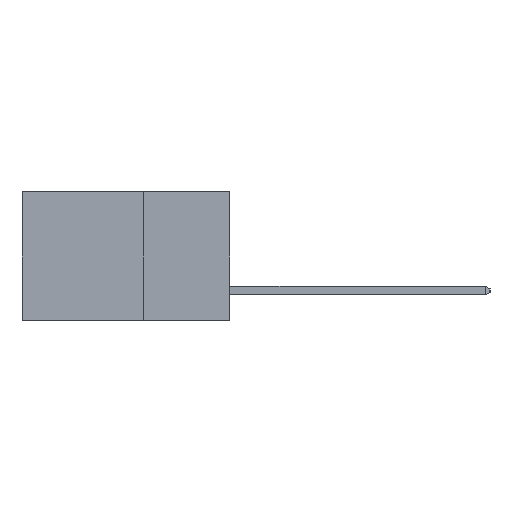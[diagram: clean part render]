
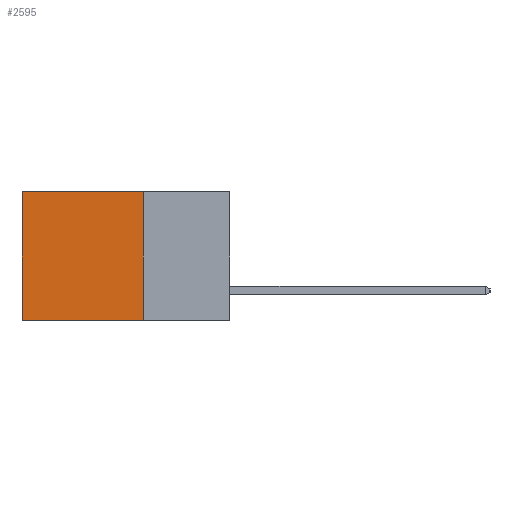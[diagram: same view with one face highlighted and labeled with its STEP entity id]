
A CAD part, left-side view. The second image highlights one B-rep face of the part: STEP entity #2595.
In plain terms, the highlighted planar face has unit normal (-1, 0, 0).
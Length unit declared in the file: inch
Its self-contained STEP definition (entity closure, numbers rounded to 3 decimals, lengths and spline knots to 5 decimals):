
#247 = EDGE_CURVE ( 'NONE', #2539, #21409, #13997, .T. ) ;
#2112 = DIRECTION ( 'NONE',  ( 0., 0., -1. ) ) ;
#2196 = CARTESIAN_POINT ( 'NONE',  ( 0.2615, 0.25, -0.37 ) ) ;
#2205 = PLANE ( 'NONE',  #9097 ) ;
#2209 = DIRECTION ( 'NONE',  ( 1., 0., 0. ) ) ;
#2308 = LINE ( 'NONE', #2196, #12201 ) ;
#2479 = CARTESIAN_POINT ( 'NONE',  ( 0.2615, 0.25, -0.37 ) ) ;
#2539 = VERTEX_POINT ( 'NONE', #4524 ) ;
#2542 = CARTESIAN_POINT ( 'NONE',  ( 0.2615, 0.25, -0.37 ) ) ;
#2595 = ADVANCED_FACE ( 'NONE', ( #17513 ), #2205, .F. ) ;
#2768 = DIRECTION ( 'NONE',  ( 0., 0., -1. ) ) ;
#3062 = DIRECTION ( 'NONE',  ( 0., 1., 0. ) ) ;
#4524 = CARTESIAN_POINT ( 'NONE',  ( 0.2615, 0.25, 0. ) ) ;
#4621 = ORIENTED_EDGE ( 'NONE', *, *, #8058, .T. ) ;
#4740 = VERTEX_POINT ( 'NONE', #10091 ) ;
#4751 = CARTESIAN_POINT ( 'NONE',  ( 0.2615, 0.25, 0. ) ) ;
#6297 = CARTESIAN_POINT ( 'NONE',  ( 0.2615, 0.6, -0.37 ) ) ;
#6882 = CARTESIAN_POINT ( 'NONE',  ( 0.2615, 0.6, 0. ) ) ;
#7228 = DIRECTION ( 'NONE',  ( 0., 0., -1. ) ) ;
#7273 = DIRECTION ( 'NONE',  ( 0., 1., 0. ) ) ;
#7472 = EDGE_CURVE ( 'NONE', #4740, #14916, #8184, .T. ) ;
#7551 = EDGE_CURVE ( 'NONE', #2539, #4740, #2308, .T. ) ;
#8058 = EDGE_CURVE ( 'NONE', #21409, #14916, #22479, .T. ) ;
#8184 = LINE ( 'NONE', #2542, #24559 ) ;
#9097 = AXIS2_PLACEMENT_3D ( 'NONE', #2479, #2209, #2112 ) ;
#10091 = CARTESIAN_POINT ( 'NONE',  ( 0.2615, 0.25, -0.37 ) ) ;
#12201 = VECTOR ( 'NONE', #2768, 39.37008 ) ;
#12480 = ORIENTED_EDGE ( 'NONE', *, *, #247, .T. ) ;
#13368 = VECTOR ( 'NONE', #7273, 39.37008 ) ;
#13997 = LINE ( 'NONE', #4751, #13368 ) ;
#14916 = VERTEX_POINT ( 'NONE', #20946 ) ;
#16014 = EDGE_LOOP ( 'NONE', ( #4621, #19154, #24870, #12480 ) ) ;
#17513 = FACE_OUTER_BOUND ( 'NONE', #16014, .T. ) ;
#19154 = ORIENTED_EDGE ( 'NONE', *, *, #7472, .F. ) ;
#20946 = CARTESIAN_POINT ( 'NONE',  ( 0.2615, 0.6, -0.37 ) ) ;
#21409 = VERTEX_POINT ( 'NONE', #6882 ) ;
#21919 = VECTOR ( 'NONE', #7228, 39.37008 ) ;
#22479 = LINE ( 'NONE', #6297, #21919 ) ;
#24559 = VECTOR ( 'NONE', #3062, 39.37008 ) ;
#24870 = ORIENTED_EDGE ( 'NONE', *, *, #7551, .F. ) ;
